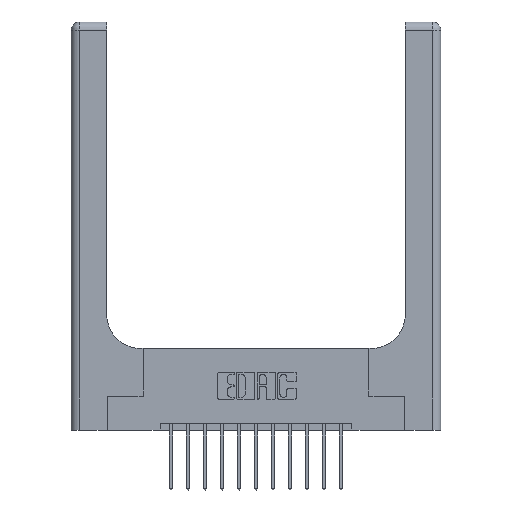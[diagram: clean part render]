
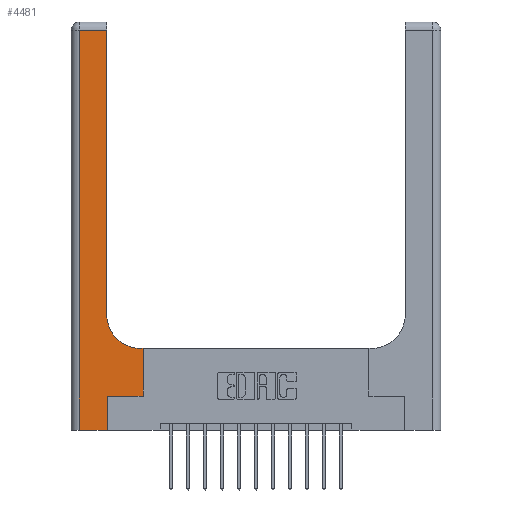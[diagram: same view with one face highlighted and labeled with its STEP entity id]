
A CAD part, top view. The second image highlights one B-rep face of the part: STEP entity #4481.
In plain terms, the highlighted planar face has unit normal (0, 0, 1).
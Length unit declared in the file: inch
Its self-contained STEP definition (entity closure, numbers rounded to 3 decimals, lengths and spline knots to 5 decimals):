
#40 = CARTESIAN_POINT ( 'NONE',  ( 0.528, 0.25, 0.37 ) ) ;
#198 = DIRECTION ( 'NONE',  ( -1., 0., 0. ) ) ;
#235 = LINE ( 'NONE', #2661, #13651 ) ;
#573 = DIRECTION ( 'NONE',  ( 0., 1., 0. ) ) ;
#689 = ORIENTED_EDGE ( 'NONE', *, *, #2076, .T. ) ;
#1146 = VERTEX_POINT ( 'NONE', #1747 ) ;
#1196 = VERTEX_POINT ( 'NONE', #9815 ) ;
#1316 = VECTOR ( 'NONE', #573, 39.37008 ) ;
#1732 = EDGE_CURVE ( 'NONE', #6815, #1146, #14723, .T. ) ;
#1747 = CARTESIAN_POINT ( 'NONE',  ( 0.06, 2.94, 0.37 ) ) ;
#1842 = CARTESIAN_POINT ( 'NONE',  ( 0.06, 0., 0.37 ) ) ;
#2076 = EDGE_CURVE ( 'NONE', #1146, #15452, #11143, .T. ) ;
#2188 = VECTOR ( 'NONE', #10503, 39.37008 ) ;
#2618 = CARTESIAN_POINT ( 'NONE',  ( 0.265, 0., 0.37 ) ) ;
#2628 = PLANE ( 'NONE',  #4705 ) ;
#2661 = CARTESIAN_POINT ( 'NONE',  ( 0.26, 0.6, 0.37 ) ) ;
#3069 = ORIENTED_EDGE ( 'NONE', *, *, #1732, .T. ) ;
#3275 = VERTEX_POINT ( 'NONE', #10979 ) ;
#3729 = CARTESIAN_POINT ( 'NONE',  ( 0.51, 0.6, 0.37 ) ) ;
#4119 = DIRECTION ( 'NONE',  ( -1., 0., 0. ) ) ;
#4442 = VECTOR ( 'NONE', #6691, 39.37008 ) ;
#4481 = ADVANCED_FACE ( 'NONE', ( #15705 ), #2628, .F. ) ;
#4517 = EDGE_CURVE ( 'NONE', #15452, #16287, #16293, .T. ) ;
#4521 = CARTESIAN_POINT ( 'NONE',  ( 0., 0., 0.37 ) ) ;
#4705 = AXIS2_PLACEMENT_3D ( 'NONE', #5308, #15869, #198 ) ;
#5105 = AXIS2_PLACEMENT_3D ( 'NONE', #7359, #12596, #14915 ) ;
#5118 = VERTEX_POINT ( 'NONE', #3729 ) ;
#5308 = CARTESIAN_POINT ( 'NONE',  ( 0., 3., 0.37 ) ) ;
#5591 = ORIENTED_EDGE ( 'NONE', *, *, #6121, .T. ) ;
#5661 = EDGE_CURVE ( 'NONE', #3275, #11090, #14522, .T. ) ;
#5952 = LINE ( 'NONE', #13674, #1316 ) ;
#6121 = EDGE_CURVE ( 'NONE', #5118, #1196, #14689, .T. ) ;
#6205 = DIRECTION ( 'NONE',  ( 0., -1., 0. ) ) ;
#6512 = LINE ( 'NONE', #2618, #14333 ) ;
#6594 = DIRECTION ( 'NONE',  ( 0., 1., 0. ) ) ;
#6691 = DIRECTION ( 'NONE',  ( 0., 1., 0. ) ) ;
#6738 = ORIENTED_EDGE ( 'NONE', *, *, #10333, .T. ) ;
#6815 = VERTEX_POINT ( 'NONE', #8063 ) ;
#7359 = CARTESIAN_POINT ( 'NONE',  ( 0.51, 0.85, 0.37 ) ) ;
#7962 = ORIENTED_EDGE ( 'NONE', *, *, #15398, .T. ) ;
#8045 = DIRECTION ( 'NONE',  ( 1., 0., 0. ) ) ;
#8051 = VECTOR ( 'NONE', #8045, 39.37008 ) ;
#8063 = CARTESIAN_POINT ( 'NONE',  ( 0.26, 2.94, 0.37 ) ) ;
#9815 = CARTESIAN_POINT ( 'NONE',  ( 0.26, 0.85, 0.37 ) ) ;
#10333 = EDGE_CURVE ( 'NONE', #14276, #5118, #235, .T. ) ;
#10356 = LINE ( 'NONE', #40, #4442 ) ;
#10503 = DIRECTION ( 'NONE',  ( -1., 0., 0. ) ) ;
#10670 = CARTESIAN_POINT ( 'NONE',  ( 0., 2.94, 0.37 ) ) ;
#10892 = ORIENTED_EDGE ( 'NONE', *, *, #5661, .T. ) ;
#10979 = CARTESIAN_POINT ( 'NONE',  ( 0.265, 0.25, 0.37 ) ) ;
#10990 = VECTOR ( 'NONE', #13376, 39.37008 ) ;
#11066 = EDGE_CURVE ( 'NONE', #1196, #6815, #5952, .T. ) ;
#11090 = VERTEX_POINT ( 'NONE', #16851 ) ;
#11143 = LINE ( 'NONE', #16406, #11853 ) ;
#11187 = ORIENTED_EDGE ( 'NONE', *, *, #4517, .T. ) ;
#11853 = VECTOR ( 'NONE', #6205, 39.37008 ) ;
#12437 = EDGE_LOOP ( 'NONE', ( #15067, #3069, #689, #11187, #14822, #10892, #7962, #6738, #5591 ) ) ;
#12476 = CARTESIAN_POINT ( 'NONE',  ( 0.265, 0., 0.37 ) ) ;
#12596 = DIRECTION ( 'NONE',  ( 0., 0., -1. ) ) ;
#12652 = CARTESIAN_POINT ( 'NONE',  ( 0.528, 0.6, 0.37 ) ) ;
#13376 = DIRECTION ( 'NONE',  ( 1., 0., 0. ) ) ;
#13651 = VECTOR ( 'NONE', #4119, 39.37008 ) ;
#13674 = CARTESIAN_POINT ( 'NONE',  ( 0.26, 3., 0.37 ) ) ;
#14276 = VERTEX_POINT ( 'NONE', #12652 ) ;
#14333 = VECTOR ( 'NONE', #6594, 39.37008 ) ;
#14522 = LINE ( 'NONE', #16990, #8051 ) ;
#14689 = CIRCLE ( 'NONE', #5105, 0.25 ) ;
#14723 = LINE ( 'NONE', #10670, #2188 ) ;
#14822 = ORIENTED_EDGE ( 'NONE', *, *, #15700, .T. ) ;
#14915 = DIRECTION ( 'NONE',  ( 1., 0., 0. ) ) ;
#15067 = ORIENTED_EDGE ( 'NONE', *, *, #11066, .T. ) ;
#15398 = EDGE_CURVE ( 'NONE', #11090, #14276, #10356, .T. ) ;
#15452 = VERTEX_POINT ( 'NONE', #1842 ) ;
#15700 = EDGE_CURVE ( 'NONE', #16287, #3275, #6512, .T. ) ;
#15705 = FACE_OUTER_BOUND ( 'NONE', #12437, .T. ) ;
#15869 = DIRECTION ( 'NONE',  ( 0., 0., -1. ) ) ;
#16287 = VERTEX_POINT ( 'NONE', #12476 ) ;
#16293 = LINE ( 'NONE', #4521, #10990 ) ;
#16406 = CARTESIAN_POINT ( 'NONE',  ( 0.06, 3., 0.37 ) ) ;
#16851 = CARTESIAN_POINT ( 'NONE',  ( 0.528, 0.25, 0.37 ) ) ;
#16990 = CARTESIAN_POINT ( 'NONE',  ( 0.265, 0.25, 0.37 ) ) ;
